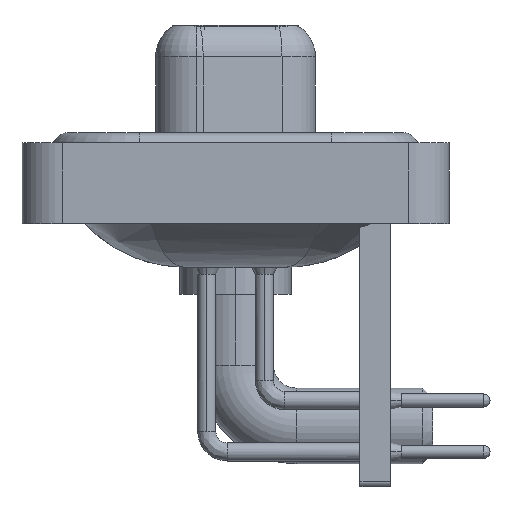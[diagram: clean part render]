
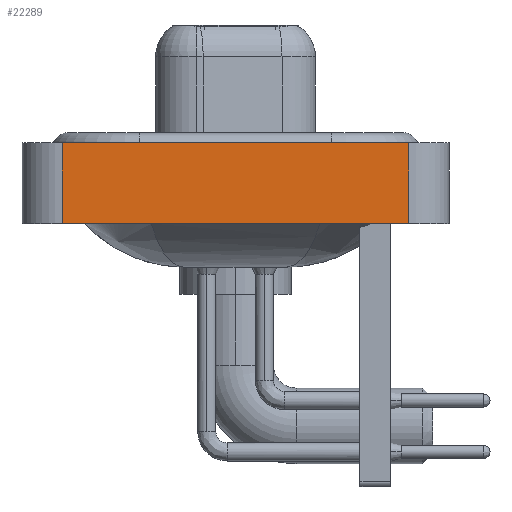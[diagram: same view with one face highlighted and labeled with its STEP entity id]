
A CAD part, left-side view. The second image highlights one B-rep face of the part: STEP entity #22289.
In plain terms, the highlighted planar face has unit normal (-1, 0, 0).
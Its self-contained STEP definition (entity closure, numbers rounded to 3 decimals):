
#321 = VECTOR ( 'NONE', #16584, 1000. ) ;
#470 = VERTEX_POINT ( 'NONE', #12501 ) ;
#538 = EDGE_CURVE ( 'NONE', #19947, #4227, #4031, .T. ) ;
#682 = DIRECTION ( 'NONE',  ( 0., 0., 1. ) ) ;
#1516 = ORIENTED_EDGE ( 'NONE', *, *, #7021, .F. ) ;
#1661 = EDGE_LOOP ( 'NONE', ( #16174, #1516, #20736, #6446 ) ) ;
#2038 = DIRECTION ( 'NONE',  ( 0., 0., 1. ) ) ;
#2126 = CARTESIAN_POINT ( 'NONE',  ( -7.3, -8.55, 0.4 ) ) ;
#2256 = DIRECTION ( 'NONE',  ( -1., 0., 0. ) ) ;
#2443 = LINE ( 'NONE', #5955, #20093 ) ;
#3450 = AXIS2_PLACEMENT_3D ( 'NONE', #12844, #2256, #2038 ) ;
#4031 = LINE ( 'NONE', #19615, #321 ) ;
#4227 = VERTEX_POINT ( 'NONE', #18773 ) ;
#4421 = CARTESIAN_POINT ( 'NONE',  ( -7.3, -8.55, 0.4 ) ) ;
#4970 = CARTESIAN_POINT ( 'NONE',  ( -7.3, 8.55, -3.6 ) ) ;
#5812 = LINE ( 'NONE', #11599, #22255 ) ;
#5955 = CARTESIAN_POINT ( 'NONE',  ( -7.3, -8.55, -3.6 ) ) ;
#6446 = ORIENTED_EDGE ( 'NONE', *, *, #538, .T. ) ;
#7021 = EDGE_CURVE ( 'NONE', #470, #16700, #11238, .T. ) ;
#7050 = EDGE_CURVE ( 'NONE', #19947, #470, #5812, .T. ) ;
#11238 = LINE ( 'NONE', #4421, #18905 ) ;
#11599 = CARTESIAN_POINT ( 'NONE',  ( -7.3, 8.55, -3.6 ) ) ;
#12501 = CARTESIAN_POINT ( 'NONE',  ( -7.3, 8.55, 0.4 ) ) ;
#12844 = CARTESIAN_POINT ( 'NONE',  ( -7.3, -8.55, -3.6 ) ) ;
#13149 = DIRECTION ( 'NONE',  ( 0., 0., 1. ) ) ;
#16174 = ORIENTED_EDGE ( 'NONE', *, *, #17372, .T. ) ;
#16582 = FACE_OUTER_BOUND ( 'NONE', #1661, .T. ) ;
#16584 = DIRECTION ( 'NONE',  ( 0., -1., 0. ) ) ;
#16700 = VERTEX_POINT ( 'NONE', #2126 ) ;
#16995 = DIRECTION ( 'NONE',  ( 0., -1., 0. ) ) ;
#17372 = EDGE_CURVE ( 'NONE', #4227, #16700, #2443, .T. ) ;
#18100 = PLANE ( 'NONE',  #3450 ) ;
#18773 = CARTESIAN_POINT ( 'NONE',  ( -7.3, -8.55, -3.6 ) ) ;
#18905 = VECTOR ( 'NONE', #16995, 1000. ) ;
#19615 = CARTESIAN_POINT ( 'NONE',  ( -7.3, -8.55, -3.6 ) ) ;
#19947 = VERTEX_POINT ( 'NONE', #4970 ) ;
#20093 = VECTOR ( 'NONE', #13149, 1000. ) ;
#20736 = ORIENTED_EDGE ( 'NONE', *, *, #7050, .F. ) ;
#22255 = VECTOR ( 'NONE', #682, 1000. ) ;
#22289 = ADVANCED_FACE ( 'NONE', ( #16582 ), #18100, .T. ) ;
